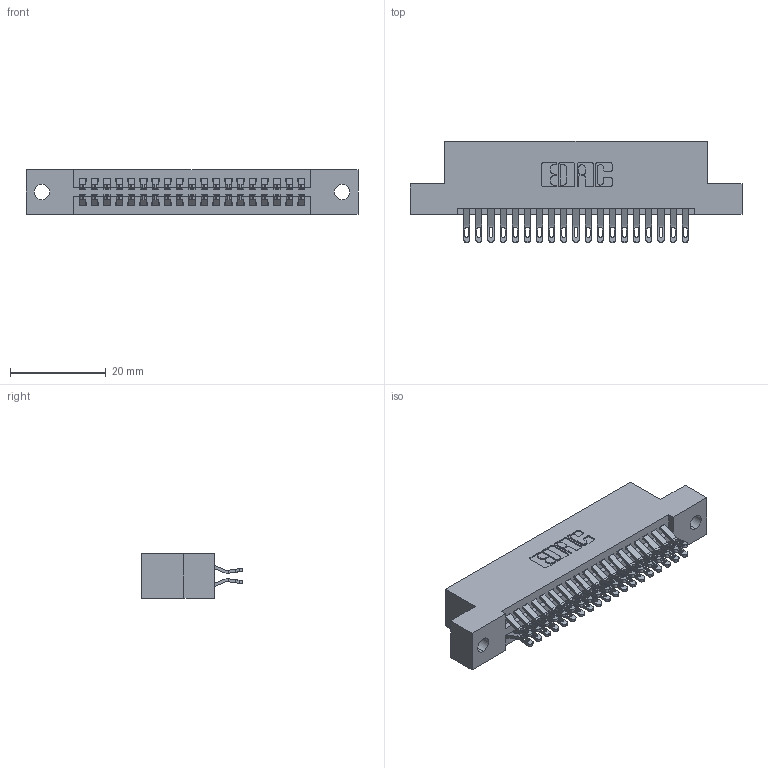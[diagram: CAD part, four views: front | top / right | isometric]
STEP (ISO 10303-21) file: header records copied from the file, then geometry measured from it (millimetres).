
FILE_DESCRIPTION (( 'STEP AP203' ), '1' );
FILE_NAME ('395-038-555-202.STEP', '2018-11-14T05:44:10', ( '' ), ( '' ), 'SwSTEP 2.0', 'SolidWorks 2016', '' );
FILE_SCHEMA (( 'CONFIG_CONTROL_DESIGN' ));
Length unit declared in the file: inch
Products named in the file (3): 345 Part_Flush Mounting Lugs - 0.128 Dia; 395-038-555-202; 345-292-001_555 Tail
Assembly tree (39 placements, depth 2):
  395-038-555-202
    345 Part_Flush Mounting Lugs - 0.128 Dia
    345-292-001_555 Tail  x38
Bounding box: 69.47 x 21.13 x 9.4 mm (x, y, z)
Volume: 6608.3 mm3; surface area: 9433.4 mm2
Topology: 39 solids, 39 shells, 2254 faces, 7067 edges, 4710 vertices
Faces by surface type: plane 1258, cylinder 996
Entity records: 18333 total; most frequent: CARTESIAN_POINT 3130, ORIENTED_EDGE 3034, DIRECTION 2757, EDGE_CURVE 1517, LINE 1289, VECTOR 1289, VERTEX_POINT 1010, AXIS2_PLACEMENT_3D 734
